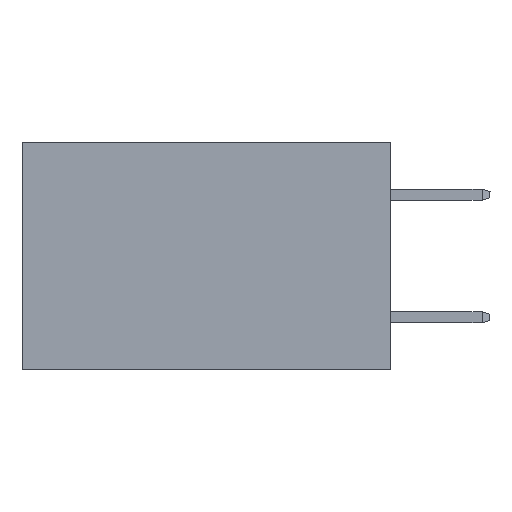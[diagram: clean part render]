
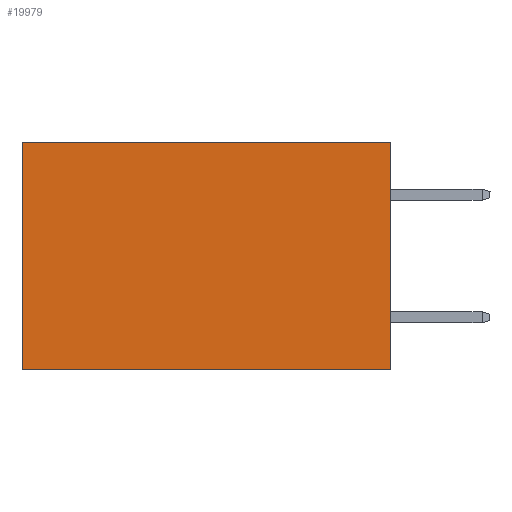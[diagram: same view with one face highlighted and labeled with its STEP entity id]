
A CAD part, left-side view. The second image highlights one B-rep face of the part: STEP entity #19979.
In plain terms, the highlighted planar face has unit normal (-1, 0, 0).
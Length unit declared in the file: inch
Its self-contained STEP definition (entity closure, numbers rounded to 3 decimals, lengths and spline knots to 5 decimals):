
#442 = CARTESIAN_POINT ( 'NONE',  ( 0.2875, 0., -0.37 ) ) ;
#725 = ORIENTED_EDGE ( 'NONE', *, *, #9097, .T. ) ;
#1052 = FACE_OUTER_BOUND ( 'NONE', #2783, .T. ) ;
#1696 = DIRECTION ( 'NONE',  ( 0., 0., -1. ) ) ;
#1995 = CARTESIAN_POINT ( 'NONE',  ( 0.2875, 0., 0. ) ) ;
#2783 = EDGE_LOOP ( 'NONE', ( #19639, #11047, #11708, #725 ) ) ;
#3016 = CARTESIAN_POINT ( 'NONE',  ( 0.2875, 0., 0. ) ) ;
#4538 = LINE ( 'NONE', #3016, #22103 ) ;
#4992 = EDGE_CURVE ( 'NONE', #21889, #7855, #20187, .T. ) ;
#6624 = VECTOR ( 'NONE', #19421, 39.37008 ) ;
#7855 = VERTEX_POINT ( 'NONE', #10048 ) ;
#7930 = LINE ( 'NONE', #11433, #16450 ) ;
#8059 = DIRECTION ( 'NONE',  ( 0., 0., -1. ) ) ;
#9097 = EDGE_CURVE ( 'NONE', #16670, #16013, #12201, .T. ) ;
#10034 = DIRECTION ( 'NONE',  ( 0., 0., -1. ) ) ;
#10048 = CARTESIAN_POINT ( 'NONE',  ( 0.2875, 0.6, -0.37 ) ) ;
#11047 = ORIENTED_EDGE ( 'NONE', *, *, #4992, .F. ) ;
#11433 = CARTESIAN_POINT ( 'NONE',  ( 0.2875, 0.6, 0. ) ) ;
#11708 = ORIENTED_EDGE ( 'NONE', *, *, #14487, .F. ) ;
#11709 = AXIS2_PLACEMENT_3D ( 'NONE', #17161, #12133, #1696 ) ;
#12133 = DIRECTION ( 'NONE',  ( 1., 0., 0. ) ) ;
#12201 = LINE ( 'NONE', #21568, #20622 ) ;
#14487 = EDGE_CURVE ( 'NONE', #16670, #21889, #4538, .T. ) ;
#16013 = VERTEX_POINT ( 'NONE', #17461 ) ;
#16450 = VECTOR ( 'NONE', #8059, 39.37008 ) ;
#16670 = VERTEX_POINT ( 'NONE', #1995 ) ;
#17161 = CARTESIAN_POINT ( 'NONE',  ( 0.2875, 0., 0. ) ) ;
#17461 = CARTESIAN_POINT ( 'NONE',  ( 0.2875, 0.6, 0. ) ) ;
#18575 = EDGE_CURVE ( 'NONE', #16013, #7855, #7930, .T. ) ;
#19248 = CARTESIAN_POINT ( 'NONE',  ( 0.2875, 0., -0.37 ) ) ;
#19421 = DIRECTION ( 'NONE',  ( 0., 1., 0. ) ) ;
#19639 = ORIENTED_EDGE ( 'NONE', *, *, #18575, .T. ) ;
#19907 = DIRECTION ( 'NONE',  ( 0., 1., 0. ) ) ;
#19979 = ADVANCED_FACE ( 'NONE', ( #1052 ), #22184, .F. ) ;
#20187 = LINE ( 'NONE', #442, #6624 ) ;
#20622 = VECTOR ( 'NONE', #19907, 39.37008 ) ;
#21568 = CARTESIAN_POINT ( 'NONE',  ( 0.2875, 0., 0. ) ) ;
#21889 = VERTEX_POINT ( 'NONE', #19248 ) ;
#22103 = VECTOR ( 'NONE', #10034, 39.37008 ) ;
#22184 = PLANE ( 'NONE',  #11709 ) ;
